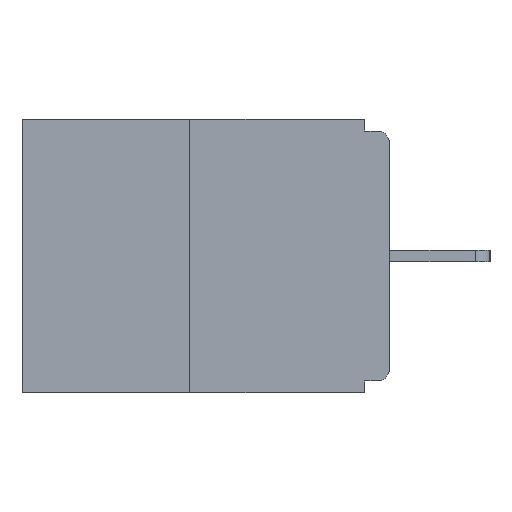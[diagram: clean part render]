
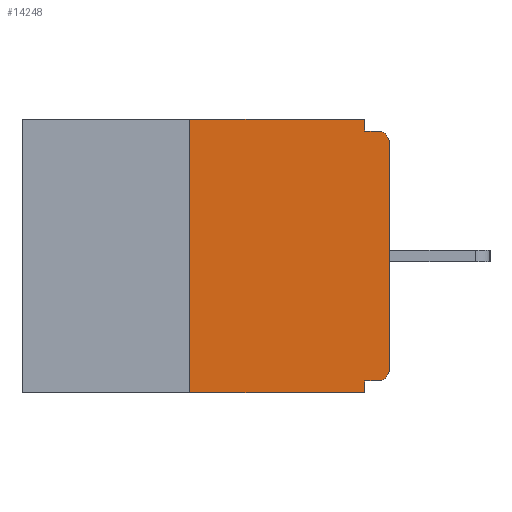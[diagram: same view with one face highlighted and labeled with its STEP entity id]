
A CAD part, left-side view. The second image highlights one B-rep face of the part: STEP entity #14248.
In plain terms, the highlighted planar face has unit normal (-1, 0, 0).
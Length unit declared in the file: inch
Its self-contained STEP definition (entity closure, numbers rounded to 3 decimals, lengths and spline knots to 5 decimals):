
#192 = DIRECTION ( 'NONE',  ( 0., -1., 0. ) ) ;
#198 = CARTESIAN_POINT ( 'NONE',  ( 0., 0.031, 0. ) ) ;
#377 = EDGE_CURVE ( 'NONE', #3066, #6169, #11389, .T. ) ;
#518 = EDGE_CURVE ( 'NONE', #5706, #20262, #5503, .T. ) ;
#708 = VERTEX_POINT ( 'NONE', #19976 ) ;
#841 = CARTESIAN_POINT ( 'NONE',  ( 0., 0.015, -0.328 ) ) ;
#1059 = EDGE_CURVE ( 'NONE', #20262, #13583, #8681, .T. ) ;
#1392 = CARTESIAN_POINT ( 'NONE',  ( 0., 0.031, -0.343 ) ) ;
#1486 = DIRECTION ( 'NONE',  ( 0., -1., 0. ) ) ;
#1701 = CARTESIAN_POINT ( 'NONE',  ( 0., 0.015, -0.03 ) ) ;
#2025 = PLANE ( 'NONE',  #10609 ) ;
#2033 = CIRCLE ( 'NONE', #12195, 0.015 ) ;
#2164 = ORIENTED_EDGE ( 'NONE', *, *, #3122, .F. ) ;
#2463 = VECTOR ( 'NONE', #15398, 39.37008 ) ;
#2947 = CARTESIAN_POINT ( 'NONE',  ( 0., 0., -0.03 ) ) ;
#3066 = VERTEX_POINT ( 'NONE', #3821 ) ;
#3122 = EDGE_CURVE ( 'NONE', #6169, #15609, #5533, .T. ) ;
#3242 = VECTOR ( 'NONE', #1486, 39.37008 ) ;
#3251 = CARTESIAN_POINT ( 'NONE',  ( 0., 0., -0.313 ) ) ;
#3569 = FACE_OUTER_BOUND ( 'NONE', #11107, .T. ) ;
#3683 = ORIENTED_EDGE ( 'NONE', *, *, #377, .F. ) ;
#3752 = CARTESIAN_POINT ( 'NONE',  ( 0., 0.031, -0.328 ) ) ;
#3821 = CARTESIAN_POINT ( 'NONE',  ( 0., 0.031, 0. ) ) ;
#3948 = EDGE_CURVE ( 'NONE', #11799, #18821, #8691, .T. ) ;
#4657 = VECTOR ( 'NONE', #7135, 39.37008 ) ;
#4787 = ORIENTED_EDGE ( 'NONE', *, *, #518, .F. ) ;
#4811 = EDGE_CURVE ( 'NONE', #18821, #15609, #2033, .T. ) ;
#5270 = DIRECTION ( 'NONE',  ( 0., 0., -1. ) ) ;
#5503 = LINE ( 'NONE', #8609, #16003 ) ;
#5533 = LINE ( 'NONE', #17979, #11538 ) ;
#5706 = VERTEX_POINT ( 'NONE', #841 ) ;
#6169 = VERTEX_POINT ( 'NONE', #16376 ) ;
#6526 = CARTESIAN_POINT ( 'NONE',  ( 0., 0.46, 0. ) ) ;
#6714 = VECTOR ( 'NONE', #192, 39.37008 ) ;
#7135 = DIRECTION ( 'NONE',  ( 0., 0., 1. ) ) ;
#7323 = CARTESIAN_POINT ( 'NONE',  ( 0., 0.015, -0.015 ) ) ;
#7367 = CARTESIAN_POINT ( 'NONE',  ( 0., 0.031, -0.343 ) ) ;
#8066 = DIRECTION ( 'NONE',  ( 0., 0., -1. ) ) ;
#8241 = EDGE_CURVE ( 'NONE', #10083, #3066, #17736, .T. ) ;
#8376 = DIRECTION ( 'NONE',  ( -1., 0., 0. ) ) ;
#8609 = CARTESIAN_POINT ( 'NONE',  ( 0., 0., -0.328 ) ) ;
#8681 = LINE ( 'NONE', #1392, #18043 ) ;
#8691 = LINE ( 'NONE', #14958, #4657 ) ;
#9946 = DIRECTION ( 'NONE',  ( 0., 0., -1. ) ) ;
#10083 = VERTEX_POINT ( 'NONE', #10561 ) ;
#10561 = CARTESIAN_POINT ( 'NONE',  ( 0., 0.25, 0. ) ) ;
#10609 = AXIS2_PLACEMENT_3D ( 'NONE', #14648, #19348, #5270 ) ;
#10864 = ORIENTED_EDGE ( 'NONE', *, *, #12603, .T. ) ;
#11107 = EDGE_LOOP ( 'NONE', ( #19823, #14707, #14073, #19292, #4787, #10864, #16738, #13812, #2164, #3683 ) ) ;
#11389 = LINE ( 'NONE', #198, #18939 ) ;
#11538 = VECTOR ( 'NONE', #18074, 39.37008 ) ;
#11799 = VERTEX_POINT ( 'NONE', #3251 ) ;
#11950 = DIRECTION ( 'NONE',  ( -1., 0., 0. ) ) ;
#12168 = DIRECTION ( 'NONE',  ( 0., 0., -1. ) ) ;
#12195 = AXIS2_PLACEMENT_3D ( 'NONE', #1701, #8376, #8066 ) ;
#12603 = EDGE_CURVE ( 'NONE', #5706, #11799, #15369, .T. ) ;
#12612 = EDGE_CURVE ( 'NONE', #708, #13583, #13701, .T. ) ;
#13583 = VERTEX_POINT ( 'NONE', #7367 ) ;
#13701 = LINE ( 'NONE', #19947, #3242 ) ;
#13812 = ORIENTED_EDGE ( 'NONE', *, *, #4811, .T. ) ;
#14073 = ORIENTED_EDGE ( 'NONE', *, *, #12612, .T. ) ;
#14248 = ADVANCED_FACE ( 'NONE', ( #3569 ), #2025, .F. ) ;
#14648 = CARTESIAN_POINT ( 'NONE',  ( 0., 0.46, 0. ) ) ;
#14707 = ORIENTED_EDGE ( 'NONE', *, *, #17056, .F. ) ;
#14958 = CARTESIAN_POINT ( 'NONE',  ( 0., 0., 0. ) ) ;
#15143 = DIRECTION ( 'NONE',  ( 0., 0., -1. ) ) ;
#15369 = CIRCLE ( 'NONE', #16334, 0.015 ) ;
#15398 = DIRECTION ( 'NONE',  ( 0., 0., 1. ) ) ;
#15609 = VERTEX_POINT ( 'NONE', #7323 ) ;
#16003 = VECTOR ( 'NONE', #18250, 39.37008 ) ;
#16334 = AXIS2_PLACEMENT_3D ( 'NONE', #19742, #11950, #15143 ) ;
#16376 = CARTESIAN_POINT ( 'NONE',  ( 0., 0.031, -0.015 ) ) ;
#16738 = ORIENTED_EDGE ( 'NONE', *, *, #3948, .T. ) ;
#17056 = EDGE_CURVE ( 'NONE', #708, #10083, #19885, .T. ) ;
#17736 = LINE ( 'NONE', #6526, #6714 ) ;
#17979 = CARTESIAN_POINT ( 'NONE',  ( 0., 0., -0.015 ) ) ;
#18043 = VECTOR ( 'NONE', #12168, 39.37008 ) ;
#18074 = DIRECTION ( 'NONE',  ( 0., -1., 0. ) ) ;
#18250 = DIRECTION ( 'NONE',  ( 0., 1., 0. ) ) ;
#18459 = CARTESIAN_POINT ( 'NONE',  ( 0., 0.25, 0. ) ) ;
#18821 = VERTEX_POINT ( 'NONE', #2947 ) ;
#18939 = VECTOR ( 'NONE', #9946, 39.37008 ) ;
#19292 = ORIENTED_EDGE ( 'NONE', *, *, #1059, .F. ) ;
#19348 = DIRECTION ( 'NONE',  ( 1., 0., 0. ) ) ;
#19742 = CARTESIAN_POINT ( 'NONE',  ( 0., 0.015, -0.313 ) ) ;
#19823 = ORIENTED_EDGE ( 'NONE', *, *, #8241, .F. ) ;
#19885 = LINE ( 'NONE', #18459, #2463 ) ;
#19947 = CARTESIAN_POINT ( 'NONE',  ( 0., 0.46, -0.343 ) ) ;
#19976 = CARTESIAN_POINT ( 'NONE',  ( 0., 0.25, -0.343 ) ) ;
#20262 = VERTEX_POINT ( 'NONE', #3752 ) ;
